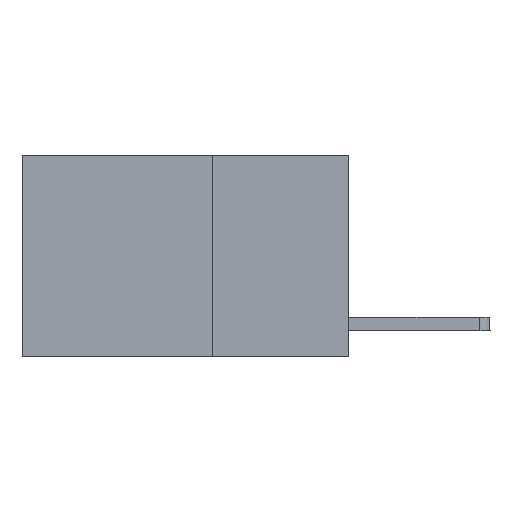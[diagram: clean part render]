
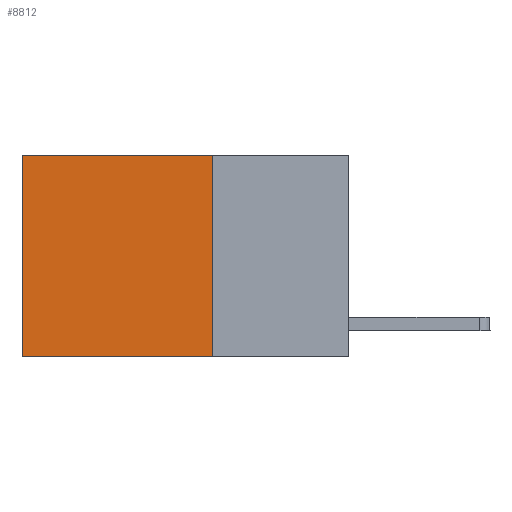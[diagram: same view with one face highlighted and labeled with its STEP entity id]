
A CAD part, left-side view. The second image highlights one B-rep face of the part: STEP entity #8812.
In plain terms, the highlighted planar face has unit normal (-1, 0, 0).
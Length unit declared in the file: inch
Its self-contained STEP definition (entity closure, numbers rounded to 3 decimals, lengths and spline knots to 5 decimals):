
#92 = PLANE ( 'NONE',  #5102 ) ;
#271 = EDGE_LOOP ( 'NONE', ( #3909, #9198, #6076, #5338 ) ) ;
#520 = DIRECTION ( 'NONE',  ( 1., 0., 0. ) ) ;
#637 = CARTESIAN_POINT ( 'NONE',  ( 0.2625, 0.25, 0. ) ) ;
#1393 = CARTESIAN_POINT ( 'NONE',  ( 0.2625, 0.25, -0.37 ) ) ;
#1489 = EDGE_CURVE ( 'NONE', #7764, #6730, #9725, .T. ) ;
#1544 = VECTOR ( 'NONE', #3155, 39.37008 ) ;
#1910 = EDGE_CURVE ( 'NONE', #2977, #7157, #2099, .T. ) ;
#2099 = LINE ( 'NONE', #6601, #6812 ) ;
#2284 = CARTESIAN_POINT ( 'NONE',  ( 0.2625, 0.25, 0. ) ) ;
#2441 = EDGE_CURVE ( 'NONE', #7764, #2977, #5281, .T. ) ;
#2844 = VECTOR ( 'NONE', #5109, 39.37008 ) ;
#2977 = VERTEX_POINT ( 'NONE', #9046 ) ;
#3133 = EDGE_CURVE ( 'NONE', #6730, #7157, #4513, .T. ) ;
#3155 = DIRECTION ( 'NONE',  ( 0., 1., 0. ) ) ;
#3646 = DIRECTION ( 'NONE',  ( 0., 1., 0. ) ) ;
#3909 = ORIENTED_EDGE ( 'NONE', *, *, #1910, .T. ) ;
#4513 = LINE ( 'NONE', #4706, #1544 ) ;
#4526 = CARTESIAN_POINT ( 'NONE',  ( 0.2625, 0.25, 0. ) ) ;
#4620 = FACE_OUTER_BOUND ( 'NONE', #271, .T. ) ;
#4706 = CARTESIAN_POINT ( 'NONE',  ( 0.2625, 0.25, -0.37 ) ) ;
#5102 = AXIS2_PLACEMENT_3D ( 'NONE', #4526, #520, #6845 ) ;
#5109 = DIRECTION ( 'NONE',  ( 0., 0., -1. ) ) ;
#5281 = LINE ( 'NONE', #637, #5716 ) ;
#5338 = ORIENTED_EDGE ( 'NONE', *, *, #2441, .T. ) ;
#5716 = VECTOR ( 'NONE', #3646, 39.37008 ) ;
#6076 = ORIENTED_EDGE ( 'NONE', *, *, #1489, .F. ) ;
#6366 = CARTESIAN_POINT ( 'NONE',  ( 0.2625, 0.25, 0. ) ) ;
#6601 = CARTESIAN_POINT ( 'NONE',  ( 0.2625, 0.6, 0. ) ) ;
#6730 = VERTEX_POINT ( 'NONE', #1393 ) ;
#6812 = VECTOR ( 'NONE', #8149, 39.37008 ) ;
#6845 = DIRECTION ( 'NONE',  ( 0., 0., -1. ) ) ;
#7157 = VERTEX_POINT ( 'NONE', #9130 ) ;
#7764 = VERTEX_POINT ( 'NONE', #6366 ) ;
#8149 = DIRECTION ( 'NONE',  ( 0., 0., -1. ) ) ;
#8812 = ADVANCED_FACE ( 'NONE', ( #4620 ), #92, .F. ) ;
#9046 = CARTESIAN_POINT ( 'NONE',  ( 0.2625, 0.6, 0. ) ) ;
#9130 = CARTESIAN_POINT ( 'NONE',  ( 0.2625, 0.6, -0.37 ) ) ;
#9198 = ORIENTED_EDGE ( 'NONE', *, *, #3133, .F. ) ;
#9725 = LINE ( 'NONE', #2284, #2844 ) ;
